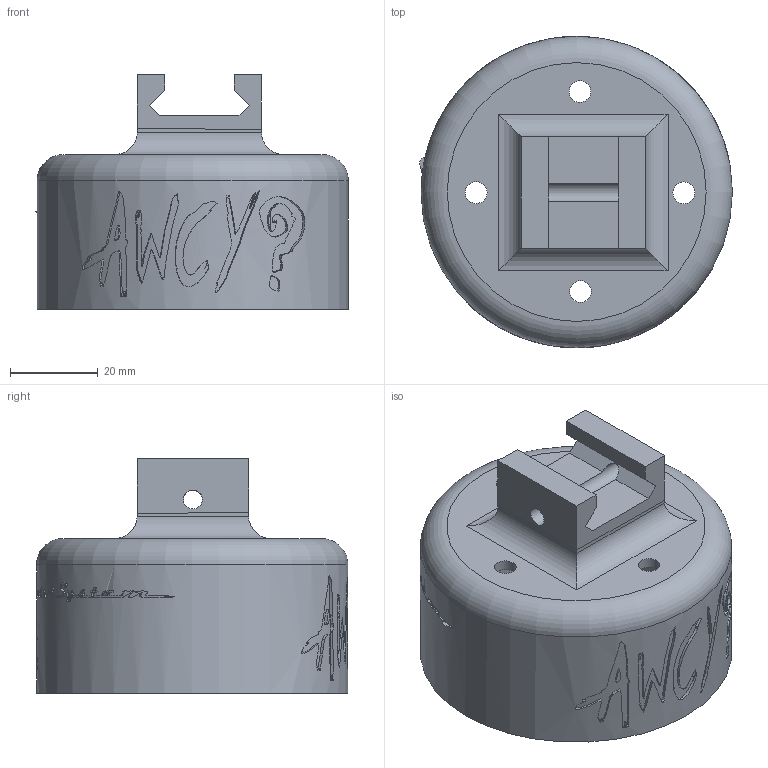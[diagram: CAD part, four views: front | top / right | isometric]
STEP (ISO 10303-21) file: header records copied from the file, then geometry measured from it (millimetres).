
FILE_DESCRIPTION(('STEP AP214'),'1');
FILE_NAME('HMB system-beer sized.stp','2021-01-18T20:18:24',(' '),(' '),'Spatial InterOp 3D',' ',' ');
FILE_SCHEMA(('AUTOMOTIVE_DESIGN { 1 0 10303 214 1 1 1 1 }'));
Length unit declared in the file: metre
Products named in the file (3): HMB system.2; Lid; HMB system-beer sized
Assembly tree (2 placements, depth 3):
  HMB system-beer sized
    HMB system.2
      Lid
Bounding box: 71.28 x 71.08 x 53.56 mm (x, y, z)
Volume: 39287.1 mm3; surface area: 25819.2 mm2
Topology: 6 solids, 7 shells, 3540 faces, 8436 edges, 4746 vertices
Faces by surface type: plane 2342, bspline 889, cone 203, cylinder 104, torus 2
Full cylindrical faces by diameter (mm): 4.3 x1, 4.962 x4, 54.876 x1, 63.32 x1, 66.348 x1, 70.964 x1
Entity records: 150994 total; most frequent: CARTESIAN_POINT 64153, ORIENTED_EDGE 15974, DIRECTION 11716, EDGE_CURVE 7987, LINE 5470, VECTOR 5470, VERTEX_POINT 4677, EDGE_LOOP 3614
